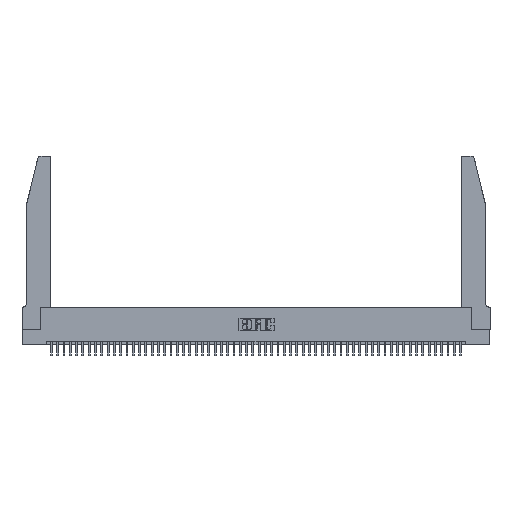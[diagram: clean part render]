
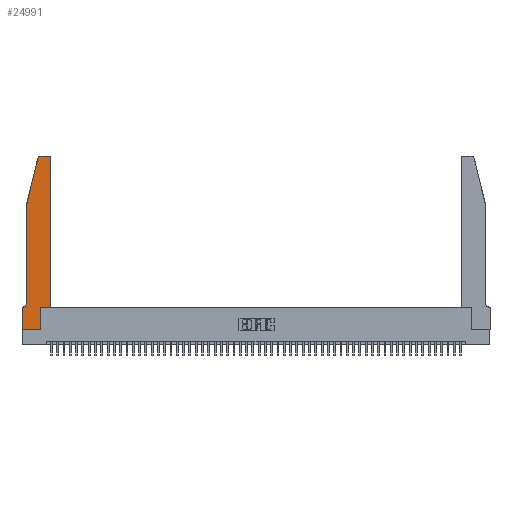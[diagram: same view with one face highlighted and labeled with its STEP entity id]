
A CAD part, top view. The second image highlights one B-rep face of the part: STEP entity #24991.
In plain terms, the highlighted planar face has unit normal (0, 0, 1).
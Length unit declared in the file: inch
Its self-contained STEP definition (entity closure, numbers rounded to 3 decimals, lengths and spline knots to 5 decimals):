
#1146 = ORIENTED_EDGE ( 'NONE', *, *, #38272, .T. ) ;
#1295 = PLANE ( 'NONE',  #44312 ) ;
#1555 = EDGE_CURVE ( 'NONE', #3986, #10554, #4281, .T. ) ;
#1743 = VECTOR ( 'NONE', #26510, 39.37008 ) ;
#1795 = DIRECTION ( 'NONE',  ( 1., 0., 0. ) ) ;
#2030 = CARTESIAN_POINT ( 'NONE',  ( 0.2865, 0.35, 0.37 ) ) ;
#2168 = CARTESIAN_POINT ( 'NONE',  ( 0.4505, 0.35, 0.37 ) ) ;
#2292 = DIRECTION ( 'NONE',  ( -1., 0., 0. ) ) ;
#3986 = VERTEX_POINT ( 'NONE', #18067 ) ;
#4281 = LINE ( 'NONE', #22855, #5573 ) ;
#4831 = CARTESIAN_POINT ( 'NONE',  ( 0.0055, 0.35, 0.37 ) ) ;
#5010 = ORIENTED_EDGE ( 'NONE', *, *, #12055, .T. ) ;
#5098 = DIRECTION ( 'NONE',  ( 1., 0., 0. ) ) ;
#5277 = DIRECTION ( 'NONE',  ( 0., 0., 1. ) ) ;
#5573 = VECTOR ( 'NONE', #47550, 39.37008 ) ;
#6532 = VERTEX_POINT ( 'NONE', #43208 ) ;
#8590 = AXIS2_PLACEMENT_3D ( 'NONE', #31497, #22861, #47912 ) ;
#8843 = ORIENTED_EDGE ( 'NONE', *, *, #9907, .T. ) ;
#9877 = DIRECTION ( 'NONE',  ( -0.239, -0.971, 0. ) ) ;
#9907 = EDGE_CURVE ( 'NONE', #21821, #41457, #17065, .T. ) ;
#10439 = CARTESIAN_POINT ( 'NONE',  ( 0.284, 2.75, 0.37 ) ) ;
#10554 = VERTEX_POINT ( 'NONE', #15746 ) ;
#10838 = ORIENTED_EDGE ( 'NONE', *, *, #41077, .T. ) ;
#12055 = EDGE_CURVE ( 'NONE', #15989, #38743, #30474, .T. ) ;
#12545 = EDGE_CURVE ( 'NONE', #6532, #17826, #22673, .T. ) ;
#12756 = LINE ( 'NONE', #43797, #1743 ) ;
#13450 = LINE ( 'NONE', #26324, #47662 ) ;
#13787 = EDGE_CURVE ( 'NONE', #17826, #30432, #52798, .T. ) ;
#14149 = CARTESIAN_POINT ( 'NONE',  ( 0.4505, 0.35, 0.37 ) ) ;
#14156 = CARTESIAN_POINT ( 'NONE',  ( 0.2865, 0.35, 0.37 ) ) ;
#15247 = ORIENTED_EDGE ( 'NONE', *, *, #35722, .T. ) ;
#15746 = CARTESIAN_POINT ( 'NONE',  ( 0.0755, 0.42, 0.37 ) ) ;
#15989 = VERTEX_POINT ( 'NONE', #10439 ) ;
#16113 = ORIENTED_EDGE ( 'NONE', *, *, #40401, .T. ) ;
#16795 = ORIENTED_EDGE ( 'NONE', *, *, #50621, .T. ) ;
#17065 = CIRCLE ( 'NONE', #8590, 0.03 ) ;
#17826 = VERTEX_POINT ( 'NONE', #24364 ) ;
#18067 = CARTESIAN_POINT ( 'NONE',  ( 0.0755, 2., 0.37 ) ) ;
#18811 = CARTESIAN_POINT ( 'NONE',  ( 0.0055, 0.42, 0.37 ) ) ;
#21357 = ORIENTED_EDGE ( 'NONE', *, *, #13787, .T. ) ;
#21821 = VERTEX_POINT ( 'NONE', #29935 ) ;
#22673 = LINE ( 'NONE', #51421, #38105 ) ;
#22855 = CARTESIAN_POINT ( 'NONE',  ( 0.0755, 2., 0.37 ) ) ;
#22861 = DIRECTION ( 'NONE',  ( 0., 0., 1. ) ) ;
#22968 = VERTEX_POINT ( 'NONE', #25176 ) ;
#23591 = CIRCLE ( 'NONE', #47297, 0.07 ) ;
#24241 = DIRECTION ( 'NONE',  ( 0., 0., 1. ) ) ;
#24364 = CARTESIAN_POINT ( 'NONE',  ( 0.2865, 0., 0.37 ) ) ;
#24631 = ORIENTED_EDGE ( 'NONE', *, *, #33402, .T. ) ;
#24991 = ADVANCED_FACE ( 'NONE', ( #30138 ), #1295, .T. ) ;
#25176 = CARTESIAN_POINT ( 'NONE',  ( 0., 0.35, 0.37 ) ) ;
#25451 = CARTESIAN_POINT ( 'NONE',  ( 0.4205, 2.75, 0.37 ) ) ;
#26324 = CARTESIAN_POINT ( 'NONE',  ( 0.0755, 2., 0.37 ) ) ;
#26510 = DIRECTION ( 'NONE',  ( 0., -1., 0. ) ) ;
#27336 = VERTEX_POINT ( 'NONE', #4831 ) ;
#29564 = VECTOR ( 'NONE', #52012, 39.37008 ) ;
#29935 = CARTESIAN_POINT ( 'NONE',  ( 0.4505, 2.72, 0.37 ) ) ;
#30077 = VECTOR ( 'NONE', #34706, 39.37008 ) ;
#30085 = AXIS2_PLACEMENT_3D ( 'NONE', #52378, #24241, #40085 ) ;
#30138 = FACE_OUTER_BOUND ( 'NONE', #32945, .T. ) ;
#30243 = EDGE_CURVE ( 'NONE', #30432, #31884, #45608, .T. ) ;
#30432 = VERTEX_POINT ( 'NONE', #2030 ) ;
#30474 = CIRCLE ( 'NONE', #30085, 0.03 ) ;
#30833 = ORIENTED_EDGE ( 'NONE', *, *, #30243, .T. ) ;
#31426 = CARTESIAN_POINT ( 'NONE',  ( 0.2605, 2.75, 0.37 ) ) ;
#31497 = CARTESIAN_POINT ( 'NONE',  ( 0.4205, 2.72, 0.37 ) ) ;
#31884 = VERTEX_POINT ( 'NONE', #34477 ) ;
#31952 = DIRECTION ( 'NONE',  ( -1., 0., 0. ) ) ;
#32945 = EDGE_LOOP ( 'NONE', ( #10838, #5010, #1146, #46492, #16795, #16113, #15247, #41026, #21357, #30833, #24631, #8843 ) ) ;
#33402 = EDGE_CURVE ( 'NONE', #31884, #21821, #50883, .T. ) ;
#34477 = CARTESIAN_POINT ( 'NONE',  ( 0.4505, 0.35, 0.37 ) ) ;
#34706 = DIRECTION ( 'NONE',  ( 1., 0., 0. ) ) ;
#35222 = VECTOR ( 'NONE', #2292, 39.37008 ) ;
#35370 = DIRECTION ( 'NONE',  ( 0., 1., 0. ) ) ;
#35722 = EDGE_CURVE ( 'NONE', #22968, #6532, #12756, .T. ) ;
#35779 = VECTOR ( 'NONE', #31952, 39.37008 ) ;
#35833 = CARTESIAN_POINT ( 'NONE',  ( 0.0755, 0.35, 0.37 ) ) ;
#38105 = VECTOR ( 'NONE', #1795, 39.37008 ) ;
#38272 = EDGE_CURVE ( 'NONE', #38743, #3986, #13450, .T. ) ;
#38743 = VERTEX_POINT ( 'NONE', #50078 ) ;
#40085 = DIRECTION ( 'NONE',  ( 1., 0., 0. ) ) ;
#40401 = EDGE_CURVE ( 'NONE', #27336, #22968, #46843, .T. ) ;
#41026 = ORIENTED_EDGE ( 'NONE', *, *, #12545, .T. ) ;
#41077 = EDGE_CURVE ( 'NONE', #41457, #15989, #42254, .T. ) ;
#41457 = VERTEX_POINT ( 'NONE', #25451 ) ;
#42254 = LINE ( 'NONE', #31426, #35779 ) ;
#43208 = CARTESIAN_POINT ( 'NONE',  ( 0., 0., 0.37 ) ) ;
#43797 = CARTESIAN_POINT ( 'NONE',  ( 0., 0., 0.37 ) ) ;
#44312 = AXIS2_PLACEMENT_3D ( 'NONE', #50214, #5277, #5098 ) ;
#45608 = LINE ( 'NONE', #14149, #30077 ) ;
#46492 = ORIENTED_EDGE ( 'NONE', *, *, #1555, .T. ) ;
#46843 = LINE ( 'NONE', #35833, #35222 ) ;
#47297 = AXIS2_PLACEMENT_3D ( 'NONE', #18811, #51278, #51810 ) ;
#47550 = DIRECTION ( 'NONE',  ( 0., -1., 0. ) ) ;
#47662 = VECTOR ( 'NONE', #9877, 39.37008 ) ;
#47912 = DIRECTION ( 'NONE',  ( 1., 0., 0. ) ) ;
#48292 = VECTOR ( 'NONE', #35370, 39.37008 ) ;
#50078 = CARTESIAN_POINT ( 'NONE',  ( 0.25487, 2.72718, 0.37 ) ) ;
#50214 = CARTESIAN_POINT ( 'NONE',  ( 0., 0.35, 0.37 ) ) ;
#50621 = EDGE_CURVE ( 'NONE', #10554, #27336, #23591, .T. ) ;
#50883 = LINE ( 'NONE', #2168, #48292 ) ;
#51278 = DIRECTION ( 'NONE',  ( 0., 0., -1. ) ) ;
#51421 = CARTESIAN_POINT ( 'NONE',  ( 0., 0., 0.37 ) ) ;
#51810 = DIRECTION ( 'NONE',  ( -1., 0., 0. ) ) ;
#52012 = DIRECTION ( 'NONE',  ( 0., 1., 0. ) ) ;
#52378 = CARTESIAN_POINT ( 'NONE',  ( 0.284, 2.72, 0.37 ) ) ;
#52798 = LINE ( 'NONE', #14156, #29564 ) ;
